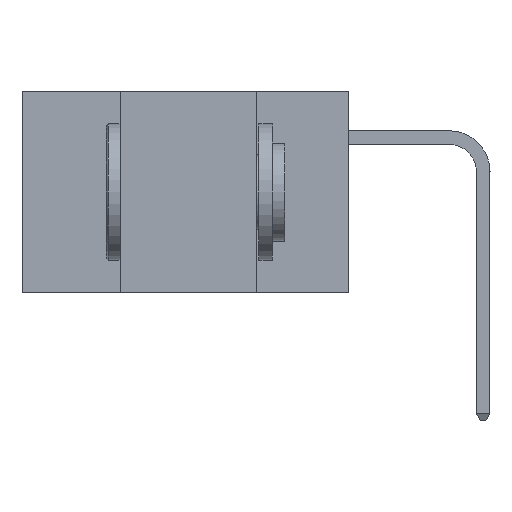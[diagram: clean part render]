
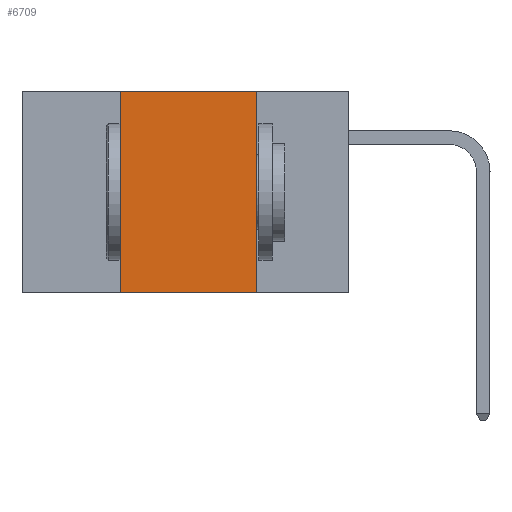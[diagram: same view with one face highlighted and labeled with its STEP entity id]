
A CAD part, left-side view. The second image highlights one B-rep face of the part: STEP entity #6709.
In plain terms, the highlighted planar face has unit normal (-1, 0, 0).
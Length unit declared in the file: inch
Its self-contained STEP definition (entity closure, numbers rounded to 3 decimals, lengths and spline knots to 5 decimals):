
#293 = DIRECTION ( 'NONE',  ( 0., -1., 0. ) ) ;
#358 = CARTESIAN_POINT ( 'NONE',  ( 0., 0.6, 0. ) ) ;
#361 = DIRECTION ( 'NONE',  ( 0., -1., 0. ) ) ;
#780 = ORIENTED_EDGE ( 'NONE', *, *, #15703, .F. ) ;
#1258 = ORIENTED_EDGE ( 'NONE', *, *, #6000, .F. ) ;
#1501 = ORIENTED_EDGE ( 'NONE', *, *, #17243, .F. ) ;
#1752 = LINE ( 'NONE', #8634, #4989 ) ;
#2816 = CARTESIAN_POINT ( 'NONE',  ( 0., 0.6, 0. ) ) ;
#3973 = CARTESIAN_POINT ( 'NONE',  ( 0., 0.17, 0. ) ) ;
#4115 = VERTEX_POINT ( 'NONE', #10791 ) ;
#4198 = DIRECTION ( 'NONE',  ( 1., 0., 0. ) ) ;
#4530 = CARTESIAN_POINT ( 'NONE',  ( 0., 0.42, -0.37 ) ) ;
#4989 = VECTOR ( 'NONE', #361, 39.37008 ) ;
#5418 = ORIENTED_EDGE ( 'NONE', *, *, #5648, .T. ) ;
#5648 = EDGE_CURVE ( 'NONE', #17239, #15575, #1752, .T. ) ;
#6000 = EDGE_CURVE ( 'NONE', #9618, #15575, #7073, .T. ) ;
#6511 = CARTESIAN_POINT ( 'NONE',  ( 0., 0.17, -0.37 ) ) ;
#6652 = VECTOR ( 'NONE', #293, 39.37008 ) ;
#6709 = ADVANCED_FACE ( 'NONE', ( #9628 ), #10998, .F. ) ;
#7073 = LINE ( 'NONE', #3973, #10329 ) ;
#8634 = CARTESIAN_POINT ( 'NONE',  ( 0., 0.6, -0.37 ) ) ;
#8942 = AXIS2_PLACEMENT_3D ( 'NONE', #2816, #4198, #13695 ) ;
#9618 = VERTEX_POINT ( 'NONE', #11480 ) ;
#9628 = FACE_OUTER_BOUND ( 'NONE', #12807, .T. ) ;
#10147 = VECTOR ( 'NONE', #13596, 39.37008 ) ;
#10329 = VECTOR ( 'NONE', #16142, 39.37008 ) ;
#10791 = CARTESIAN_POINT ( 'NONE',  ( 0., 0.42, 0. ) ) ;
#10998 = PLANE ( 'NONE',  #8942 ) ;
#11480 = CARTESIAN_POINT ( 'NONE',  ( 0., 0.17, 0. ) ) ;
#12234 = CARTESIAN_POINT ( 'NONE',  ( 0., 0.42, 0. ) ) ;
#12807 = EDGE_LOOP ( 'NONE', ( #1258, #1501, #780, #5418 ) ) ;
#13596 = DIRECTION ( 'NONE',  ( 0., 0., 1. ) ) ;
#13695 = DIRECTION ( 'NONE',  ( 0., 0., -1. ) ) ;
#13875 = LINE ( 'NONE', #358, #6652 ) ;
#14122 = LINE ( 'NONE', #12234, #10147 ) ;
#15575 = VERTEX_POINT ( 'NONE', #6511 ) ;
#15703 = EDGE_CURVE ( 'NONE', #17239, #4115, #14122, .T. ) ;
#16142 = DIRECTION ( 'NONE',  ( 0., 0., -1. ) ) ;
#17239 = VERTEX_POINT ( 'NONE', #4530 ) ;
#17243 = EDGE_CURVE ( 'NONE', #4115, #9618, #13875, .T. ) ;
